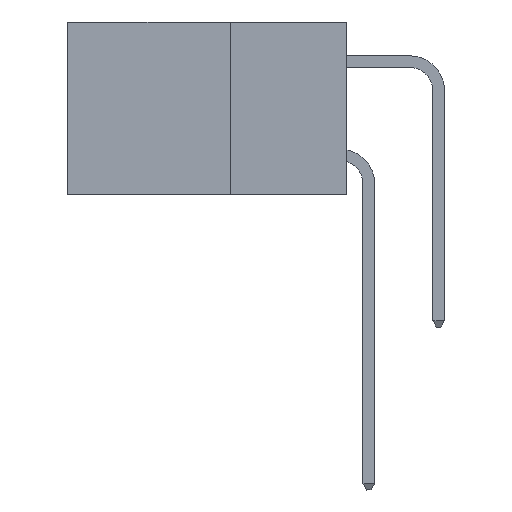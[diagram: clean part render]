
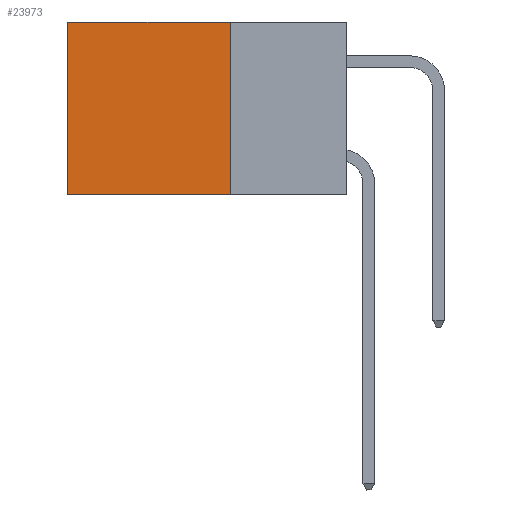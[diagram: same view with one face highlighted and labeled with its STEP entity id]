
A CAD part, left-side view. The second image highlights one B-rep face of the part: STEP entity #23973.
In plain terms, the highlighted planar face has unit normal (-1, 0, 0).
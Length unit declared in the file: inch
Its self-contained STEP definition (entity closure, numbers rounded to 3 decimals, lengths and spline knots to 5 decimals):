
#1311 = VECTOR ( 'NONE', #32806, 39.37008 ) ;
#1805 = VECTOR ( 'NONE', #35671, 39.37008 ) ;
#2459 = FACE_OUTER_BOUND ( 'NONE', #37408, .T. ) ;
#4870 = CARTESIAN_POINT ( 'NONE',  ( 0.2875, 0.6, -0.37 ) ) ;
#5530 = LINE ( 'NONE', #6044, #1805 ) ;
#5767 = CARTESIAN_POINT ( 'NONE',  ( 0.2875, 0.25, -0.37 ) ) ;
#6044 = CARTESIAN_POINT ( 'NONE',  ( 0.2875, 0.25, 0. ) ) ;
#6805 = CARTESIAN_POINT ( 'NONE',  ( 0.2875, 0.6, 0. ) ) ;
#7261 = VERTEX_POINT ( 'NONE', #28166 ) ;
#9223 = LINE ( 'NONE', #5767, #1311 ) ;
#9459 = DIRECTION ( 'NONE',  ( 0., 0., -1. ) ) ;
#9515 = ORIENTED_EDGE ( 'NONE', *, *, #12130, .T. ) ;
#10348 = DIRECTION ( 'NONE',  ( 0., 0., -1. ) ) ;
#12130 = EDGE_CURVE ( 'NONE', #7261, #26378, #29608, .T. ) ;
#15377 = EDGE_CURVE ( 'NONE', #26378, #22563, #37413, .T. ) ;
#15781 = DIRECTION ( 'NONE',  ( 0., 1., 0. ) ) ;
#16585 = CARTESIAN_POINT ( 'NONE',  ( 0.2875, 0.25, 0. ) ) ;
#16740 = CARTESIAN_POINT ( 'NONE',  ( 0.2875, 0.25, 0. ) ) ;
#17926 = VERTEX_POINT ( 'NONE', #22280 ) ;
#18664 = PLANE ( 'NONE',  #32797 ) ;
#19353 = VECTOR ( 'NONE', #15781, 39.37008 ) ;
#20439 = EDGE_CURVE ( 'NONE', #17926, #22563, #9223, .T. ) ;
#21245 = DIRECTION ( 'NONE',  ( 1., 0., 0. ) ) ;
#22280 = CARTESIAN_POINT ( 'NONE',  ( 0.2875, 0.25, -0.37 ) ) ;
#22563 = VERTEX_POINT ( 'NONE', #4870 ) ;
#22932 = CARTESIAN_POINT ( 'NONE',  ( 0.2875, 0.6, 0. ) ) ;
#23973 = ADVANCED_FACE ( 'NONE', ( #2459 ), #18664, .F. ) ;
#25729 = ORIENTED_EDGE ( 'NONE', *, *, #15377, .T. ) ;
#25790 = ORIENTED_EDGE ( 'NONE', *, *, #20439, .F. ) ;
#26378 = VERTEX_POINT ( 'NONE', #6805 ) ;
#28166 = CARTESIAN_POINT ( 'NONE',  ( 0.2875, 0.25, 0. ) ) ;
#29608 = LINE ( 'NONE', #16740, #19353 ) ;
#30958 = EDGE_CURVE ( 'NONE', #7261, #17926, #5530, .T. ) ;
#32495 = ORIENTED_EDGE ( 'NONE', *, *, #30958, .F. ) ;
#32797 = AXIS2_PLACEMENT_3D ( 'NONE', #16585, #21245, #10348 ) ;
#32806 = DIRECTION ( 'NONE',  ( 0., 1., 0. ) ) ;
#35671 = DIRECTION ( 'NONE',  ( 0., 0., -1. ) ) ;
#36435 = VECTOR ( 'NONE', #9459, 39.37008 ) ;
#37408 = EDGE_LOOP ( 'NONE', ( #25729, #25790, #32495, #9515 ) ) ;
#37413 = LINE ( 'NONE', #22932, #36435 ) ;
